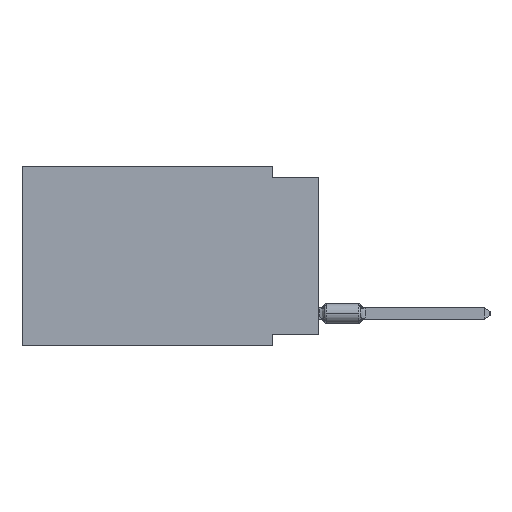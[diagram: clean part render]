
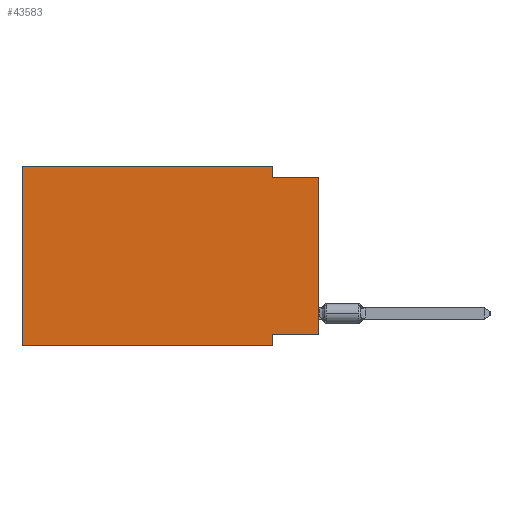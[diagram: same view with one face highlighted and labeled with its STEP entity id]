
A CAD part, left-side view. The second image highlights one B-rep face of the part: STEP entity #43583.
In plain terms, the highlighted planar face has unit normal (-1, 0, 0).
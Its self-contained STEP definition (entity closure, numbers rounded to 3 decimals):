
#986 = EDGE_CURVE ( 'NONE', #18568, #1209, #50726, .T. ) ;
#1209 = VERTEX_POINT ( 'NONE', #37437 ) ;
#2824 = LINE ( 'NONE', #18513, #51361 ) ;
#3751 = CARTESIAN_POINT ( 'NONE',  ( 0., 2.54, -9.906 ) ) ;
#4115 = ORIENTED_EDGE ( 'NONE', *, *, #16980, .T. ) ;
#5314 = DIRECTION ( 'NONE',  ( 0., 0., 1. ) ) ;
#5650 = DIRECTION ( 'NONE',  ( 0., 0., -1. ) ) ;
#7049 = EDGE_CURVE ( 'NONE', #1209, #12129, #51968, .T. ) ;
#9378 = PLANE ( 'NONE',  #10044 ) ;
#9811 = LINE ( 'NONE', #42484, #17570 ) ;
#10044 = AXIS2_PLACEMENT_3D ( 'NONE', #33830, #46008, #5650 ) ;
#12024 = VERTEX_POINT ( 'NONE', #31196 ) ;
#12129 = VERTEX_POINT ( 'NONE', #24980 ) ;
#12462 = LINE ( 'NONE', #48332, #24233 ) ;
#12932 = VERTEX_POINT ( 'NONE', #21506 ) ;
#14338 = CARTESIAN_POINT ( 'NONE',  ( 0., 16.383, 0. ) ) ;
#14780 = DIRECTION ( 'NONE',  ( 0., 0., -1. ) ) ;
#15620 = VECTOR ( 'NONE', #25389, 1000. ) ;
#16518 = CARTESIAN_POINT ( 'NONE',  ( 0., 0., -0.635 ) ) ;
#16980 = EDGE_CURVE ( 'NONE', #18568, #44281, #32602, .T. ) ;
#17568 = ORIENTED_EDGE ( 'NONE', *, *, #986, .F. ) ;
#17570 = VECTOR ( 'NONE', #5314, 1000. ) ;
#18068 = EDGE_CURVE ( 'NONE', #12024, #31929, #12462, .T. ) ;
#18513 = CARTESIAN_POINT ( 'NONE',  ( 0., 2.54, -9.906 ) ) ;
#18568 = VERTEX_POINT ( 'NONE', #44302 ) ;
#20342 = LINE ( 'NONE', #21128, #15620 ) ;
#20598 = VECTOR ( 'NONE', #32725, 1000. ) ;
#21128 = CARTESIAN_POINT ( 'NONE',  ( 0., 2.54, 0. ) ) ;
#21263 = CARTESIAN_POINT ( 'NONE',  ( 0., 2.54, -9.271 ) ) ;
#21506 = CARTESIAN_POINT ( 'NONE',  ( 0., 2.54, -0.635 ) ) ;
#21798 = VECTOR ( 'NONE', #51429, 1000. ) ;
#24233 = VECTOR ( 'NONE', #35895, 1000. ) ;
#24980 = CARTESIAN_POINT ( 'NONE',  ( 0., 2.54, 0. ) ) ;
#25389 = DIRECTION ( 'NONE',  ( 0., 0., -1. ) ) ;
#25931 = ORIENTED_EDGE ( 'NONE', *, *, #18068, .F. ) ;
#26908 = EDGE_CURVE ( 'NONE', #12932, #41918, #44932, .T. ) ;
#27942 = ORIENTED_EDGE ( 'NONE', *, *, #7049, .F. ) ;
#28588 = ORIENTED_EDGE ( 'NONE', *, *, #46377, .F. ) ;
#29846 = FACE_OUTER_BOUND ( 'NONE', #43493, .T. ) ;
#29998 = ORIENTED_EDGE ( 'NONE', *, *, #49337, .F. ) ;
#31196 = CARTESIAN_POINT ( 'NONE',  ( 0., 0., -9.271 ) ) ;
#31929 = VERTEX_POINT ( 'NONE', #21263 ) ;
#32356 = DIRECTION ( 'NONE',  ( 0., -1., 0. ) ) ;
#32602 = LINE ( 'NONE', #48760, #51161 ) ;
#32666 = VECTOR ( 'NONE', #46219, 1000. ) ;
#32725 = DIRECTION ( 'NONE',  ( 0., -1., 0. ) ) ;
#32979 = ORIENTED_EDGE ( 'NONE', *, *, #42340, .T. ) ;
#33600 = CARTESIAN_POINT ( 'NONE',  ( 0., 0., -0.635 ) ) ;
#33830 = CARTESIAN_POINT ( 'NONE',  ( 0., 16.383, 0. ) ) ;
#35895 = DIRECTION ( 'NONE',  ( 0., 1., 0. ) ) ;
#37437 = CARTESIAN_POINT ( 'NONE',  ( 0., 16.383, 0. ) ) ;
#40861 = ORIENTED_EDGE ( 'NONE', *, *, #26908, .F. ) ;
#41918 = VERTEX_POINT ( 'NONE', #33600 ) ;
#42340 = EDGE_CURVE ( 'NONE', #12024, #41918, #9811, .T. ) ;
#42484 = CARTESIAN_POINT ( 'NONE',  ( 0., 0., 0. ) ) ;
#43493 = EDGE_LOOP ( 'NONE', ( #32979, #40861, #28588, #27942, #17568, #4115, #29998, #25931 ) ) ;
#43583 = ADVANCED_FACE ( 'NONE', ( #29846 ), #9378, .F. ) ;
#44281 = VERTEX_POINT ( 'NONE', #3751 ) ;
#44302 = CARTESIAN_POINT ( 'NONE',  ( 0., 16.383, -9.906 ) ) ;
#44511 = CARTESIAN_POINT ( 'NONE',  ( 0., 16.383, 0. ) ) ;
#44932 = LINE ( 'NONE', #16518, #20598 ) ;
#46008 = DIRECTION ( 'NONE',  ( 1., 0., 0. ) ) ;
#46219 = DIRECTION ( 'NONE',  ( 0., 0., 1. ) ) ;
#46377 = EDGE_CURVE ( 'NONE', #12129, #12932, #20342, .T. ) ;
#48332 = CARTESIAN_POINT ( 'NONE',  ( 0., 0., -9.271 ) ) ;
#48760 = CARTESIAN_POINT ( 'NONE',  ( 0., 16.383, -9.906 ) ) ;
#49337 = EDGE_CURVE ( 'NONE', #31929, #44281, #2824, .T. ) ;
#50726 = LINE ( 'NONE', #14338, #32666 ) ;
#51161 = VECTOR ( 'NONE', #32356, 1000. ) ;
#51361 = VECTOR ( 'NONE', #14780, 1000. ) ;
#51429 = DIRECTION ( 'NONE',  ( 0., -1., 0. ) ) ;
#51968 = LINE ( 'NONE', #44511, #21798 ) ;
